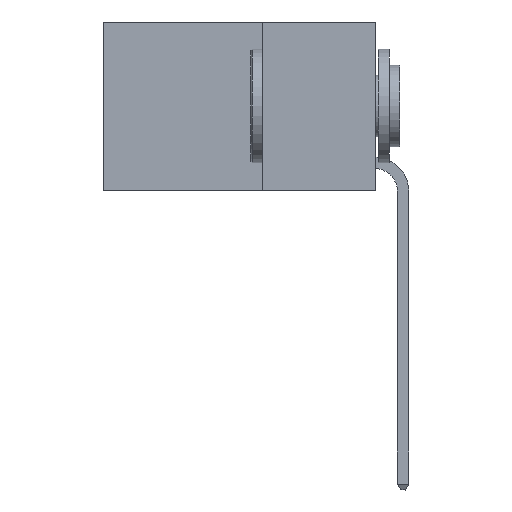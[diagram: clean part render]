
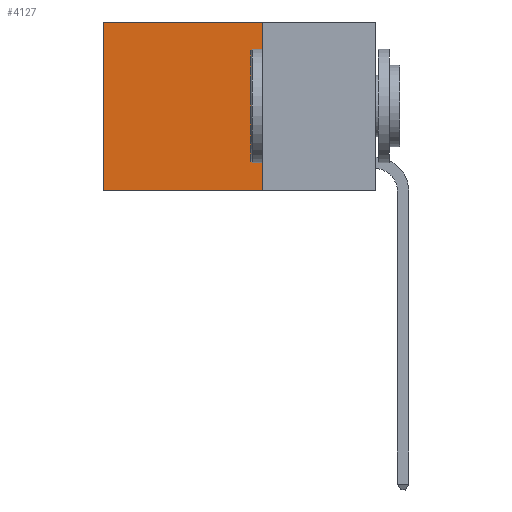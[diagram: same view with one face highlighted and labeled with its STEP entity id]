
A CAD part, left-side view. The second image highlights one B-rep face of the part: STEP entity #4127.
In plain terms, the highlighted planar face has unit normal (-1, 0, 0).
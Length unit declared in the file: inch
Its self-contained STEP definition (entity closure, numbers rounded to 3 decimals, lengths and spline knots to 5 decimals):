
#105 = EDGE_LOOP ( 'NONE', ( #1153, #1288, #1551, #1659 ) ) ;
#124 = DIRECTION ( 'NONE',  ( 0., 0., -1. ) ) ;
#173 = PLANE ( 'NONE',  #3441 ) ;
#325 = VERTEX_POINT ( 'NONE', #5936 ) ;
#603 = DIRECTION ( 'NONE',  ( 0., 1., 0. ) ) ;
#805 = CARTESIAN_POINT ( 'NONE',  ( 0.2625, 0.6, 0. ) ) ;
#977 = DIRECTION ( 'NONE',  ( 0., 0., -1. ) ) ;
#1153 = ORIENTED_EDGE ( 'NONE', *, *, #3634, .T. ) ;
#1288 = ORIENTED_EDGE ( 'NONE', *, *, #3883, .F. ) ;
#1324 = LINE ( 'NONE', #8666, #6549 ) ;
#1551 = ORIENTED_EDGE ( 'NONE', *, *, #3469, .F. ) ;
#1659 = ORIENTED_EDGE ( 'NONE', *, *, #6637, .T. ) ;
#1745 = FACE_OUTER_BOUND ( 'NONE', #105, .T. ) ;
#2057 = VERTEX_POINT ( 'NONE', #6344 ) ;
#2205 = VECTOR ( 'NONE', #3269, 39.37008 ) ;
#2426 = CARTESIAN_POINT ( 'NONE',  ( 0.2625, 0.25, 0. ) ) ;
#3269 = DIRECTION ( 'NONE',  ( 0., 0., -1. ) ) ;
#3441 = AXIS2_PLACEMENT_3D ( 'NONE', #2426, #5113, #977 ) ;
#3469 = EDGE_CURVE ( 'NONE', #7969, #325, #3540, .T. ) ;
#3540 = LINE ( 'NONE', #8310, #8501 ) ;
#3634 = EDGE_CURVE ( 'NONE', #6865, #2057, #7511, .T. ) ;
#3883 = EDGE_CURVE ( 'NONE', #325, #2057, #4143, .T. ) ;
#4127 = ADVANCED_FACE ( 'NONE', ( #1745 ), #173, .F. ) ;
#4143 = LINE ( 'NONE', #5473, #5882 ) ;
#4147 = DIRECTION ( 'NONE',  ( 0., 1., 0. ) ) ;
#4558 = CARTESIAN_POINT ( 'NONE',  ( 0.2625, 0.6, 0. ) ) ;
#5113 = DIRECTION ( 'NONE',  ( 1., 0., 0. ) ) ;
#5473 = CARTESIAN_POINT ( 'NONE',  ( 0.2625, 0.25, -0.37 ) ) ;
#5737 = CARTESIAN_POINT ( 'NONE',  ( 0.2625, 0.25, 0. ) ) ;
#5882 = VECTOR ( 'NONE', #603, 39.37008 ) ;
#5936 = CARTESIAN_POINT ( 'NONE',  ( 0.2625, 0.25, -0.37 ) ) ;
#6344 = CARTESIAN_POINT ( 'NONE',  ( 0.2625, 0.6, -0.37 ) ) ;
#6549 = VECTOR ( 'NONE', #4147, 39.37008 ) ;
#6637 = EDGE_CURVE ( 'NONE', #7969, #6865, #1324, .T. ) ;
#6865 = VERTEX_POINT ( 'NONE', #805 ) ;
#7511 = LINE ( 'NONE', #4558, #2205 ) ;
#7969 = VERTEX_POINT ( 'NONE', #5737 ) ;
#8310 = CARTESIAN_POINT ( 'NONE',  ( 0.2625, 0.25, 0. ) ) ;
#8501 = VECTOR ( 'NONE', #124, 39.37008 ) ;
#8666 = CARTESIAN_POINT ( 'NONE',  ( 0.2625, 0.25, 0. ) ) ;
